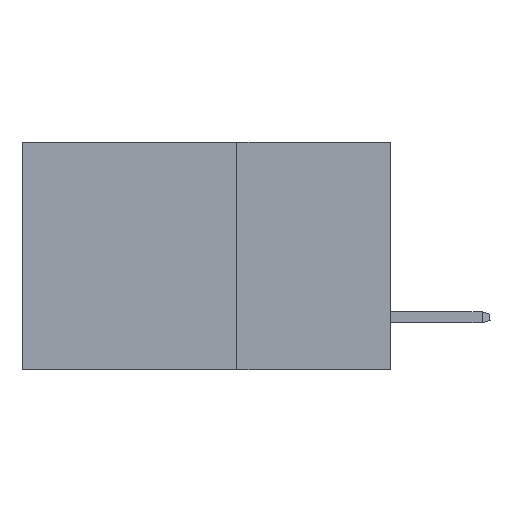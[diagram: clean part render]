
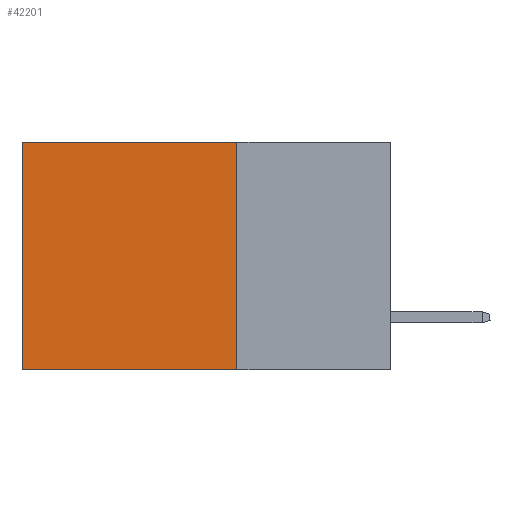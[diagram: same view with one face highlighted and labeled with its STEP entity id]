
A CAD part, left-side view. The second image highlights one B-rep face of the part: STEP entity #42201.
In plain terms, the highlighted planar face has unit normal (-1, 0, 0).
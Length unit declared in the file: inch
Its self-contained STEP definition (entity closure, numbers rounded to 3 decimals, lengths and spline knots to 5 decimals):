
#139 = VERTEX_POINT ( 'NONE', #329 ) ;
#288 = CARTESIAN_POINT ( 'NONE',  ( 0.2875, 0.25, -0.37 ) ) ;
#329 = CARTESIAN_POINT ( 'NONE',  ( 0.2875, 0.25, -0.37 ) ) ;
#640 = DIRECTION ( 'NONE',  ( 1., 0., 0. ) ) ;
#1159 = DIRECTION ( 'NONE',  ( 0., 1., 0. ) ) ;
#3533 = VERTEX_POINT ( 'NONE', #20112 ) ;
#3889 = EDGE_CURVE ( 'NONE', #33486, #3533, #32932, .T. ) ;
#4446 = ORIENTED_EDGE ( 'NONE', *, *, #3889, .T. ) ;
#5618 = EDGE_LOOP ( 'NONE', ( #4446, #33333, #14955, #40055 ) ) ;
#6202 = CARTESIAN_POINT ( 'NONE',  ( 0.2875, 0.6, 0. ) ) ;
#7136 = VECTOR ( 'NONE', #41848, 39.37008 ) ;
#7193 = AXIS2_PLACEMENT_3D ( 'NONE', #21301, #640, #24773 ) ;
#7217 = FACE_OUTER_BOUND ( 'NONE', #5618, .T. ) ;
#11173 = PLANE ( 'NONE',  #7193 ) ;
#12425 = DIRECTION ( 'NONE',  ( 0., 0., -1. ) ) ;
#13139 = VERTEX_POINT ( 'NONE', #25933 ) ;
#14674 = VECTOR ( 'NONE', #1159, 39.37008 ) ;
#14955 = ORIENTED_EDGE ( 'NONE', *, *, #28600, .F. ) ;
#16844 = LINE ( 'NONE', #39119, #14674 ) ;
#19071 = CARTESIAN_POINT ( 'NONE',  ( 0.2875, 0.25, 0. ) ) ;
#19745 = EDGE_CURVE ( 'NONE', #13139, #33486, #16844, .T. ) ;
#20112 = CARTESIAN_POINT ( 'NONE',  ( 0.2875, 0.6, -0.37 ) ) ;
#21301 = CARTESIAN_POINT ( 'NONE',  ( 0.2875, 0.25, 0. ) ) ;
#24773 = DIRECTION ( 'NONE',  ( 0., 0., -1. ) ) ;
#24998 = LINE ( 'NONE', #288, #7136 ) ;
#25933 = CARTESIAN_POINT ( 'NONE',  ( 0.2875, 0.25, 0. ) ) ;
#27566 = VECTOR ( 'NONE', #41465, 39.37008 ) ;
#28600 = EDGE_CURVE ( 'NONE', #13139, #139, #44386, .T. ) ;
#29841 = VECTOR ( 'NONE', #12425, 39.37008 ) ;
#32932 = LINE ( 'NONE', #34378, #27566 ) ;
#33333 = ORIENTED_EDGE ( 'NONE', *, *, #42744, .F. ) ;
#33486 = VERTEX_POINT ( 'NONE', #6202 ) ;
#34378 = CARTESIAN_POINT ( 'NONE',  ( 0.2875, 0.6, 0. ) ) ;
#39119 = CARTESIAN_POINT ( 'NONE',  ( 0.2875, 0.25, 0. ) ) ;
#40055 = ORIENTED_EDGE ( 'NONE', *, *, #19745, .T. ) ;
#41465 = DIRECTION ( 'NONE',  ( 0., 0., -1. ) ) ;
#41848 = DIRECTION ( 'NONE',  ( 0., 1., 0. ) ) ;
#42201 = ADVANCED_FACE ( 'NONE', ( #7217 ), #11173, .F. ) ;
#42744 = EDGE_CURVE ( 'NONE', #139, #3533, #24998, .T. ) ;
#44386 = LINE ( 'NONE', #19071, #29841 ) ;
